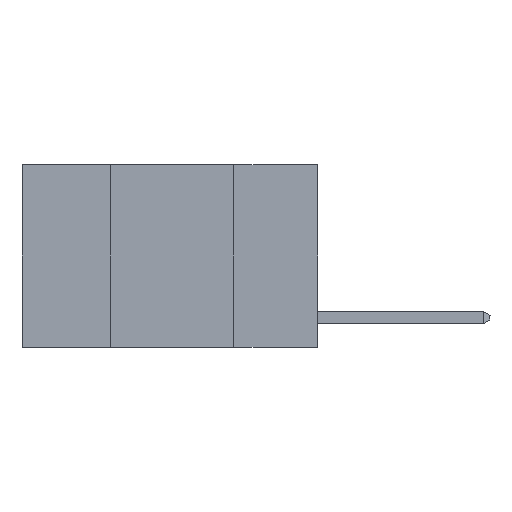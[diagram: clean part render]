
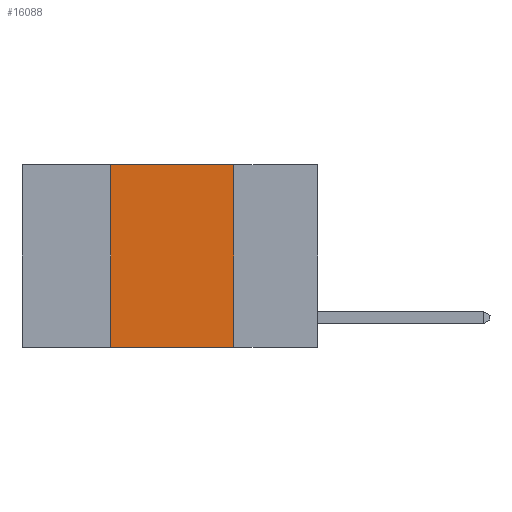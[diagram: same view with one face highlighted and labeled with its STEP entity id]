
A CAD part, left-side view. The second image highlights one B-rep face of the part: STEP entity #16088.
In plain terms, the highlighted planar face has unit normal (-1, 0, 0).
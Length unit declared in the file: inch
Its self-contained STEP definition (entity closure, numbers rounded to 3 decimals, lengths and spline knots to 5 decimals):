
#595 = DIRECTION ( 'NONE',  ( 0., -1., 0. ) ) ;
#1107 = VECTOR ( 'NONE', #4301, 39.37008 ) ;
#1128 = VERTEX_POINT ( 'NONE', #12029 ) ;
#1231 = DIRECTION ( 'NONE',  ( 0., 0., -1. ) ) ;
#1541 = CARTESIAN_POINT ( 'NONE',  ( 0., 0.6, -0.37 ) ) ;
#3491 = AXIS2_PLACEMENT_3D ( 'NONE', #14970, #16253, #1231 ) ;
#4046 = VECTOR ( 'NONE', #595, 39.37008 ) ;
#4301 = DIRECTION ( 'NONE',  ( 0., -1., 0. ) ) ;
#4798 = EDGE_CURVE ( 'NONE', #1128, #5580, #16467, .T. ) ;
#5580 = VERTEX_POINT ( 'NONE', #16965 ) ;
#5707 = EDGE_LOOP ( 'NONE', ( #5910, #8262, #6669, #9400 ) ) ;
#5910 = ORIENTED_EDGE ( 'NONE', *, *, #11385, .F. ) ;
#6521 = DIRECTION ( 'NONE',  ( 0., 0., -1. ) ) ;
#6669 = ORIENTED_EDGE ( 'NONE', *, *, #17532, .F. ) ;
#7467 = LINE ( 'NONE', #8719, #4046 ) ;
#8262 = ORIENTED_EDGE ( 'NONE', *, *, #10761, .F. ) ;
#8719 = CARTESIAN_POINT ( 'NONE',  ( 0., 0.6, 0. ) ) ;
#9289 = CARTESIAN_POINT ( 'NONE',  ( 0., 0.17, 0. ) ) ;
#9400 = ORIENTED_EDGE ( 'NONE', *, *, #4798, .T. ) ;
#10001 = VERTEX_POINT ( 'NONE', #9289 ) ;
#10712 = VERTEX_POINT ( 'NONE', #10860 ) ;
#10761 = EDGE_CURVE ( 'NONE', #10712, #10001, #7467, .T. ) ;
#10860 = CARTESIAN_POINT ( 'NONE',  ( 0., 0.42, 0. ) ) ;
#10956 = FACE_OUTER_BOUND ( 'NONE', #5707, .T. ) ;
#11385 = EDGE_CURVE ( 'NONE', #10001, #5580, #11816, .T. ) ;
#11816 = LINE ( 'NONE', #17541, #15195 ) ;
#12029 = CARTESIAN_POINT ( 'NONE',  ( 0., 0.42, -0.37 ) ) ;
#12073 = CARTESIAN_POINT ( 'NONE',  ( 0., 0.42, 0. ) ) ;
#13455 = PLANE ( 'NONE',  #3491 ) ;
#13484 = DIRECTION ( 'NONE',  ( 0., 0., 1. ) ) ;
#14899 = VECTOR ( 'NONE', #13484, 39.37008 ) ;
#14970 = CARTESIAN_POINT ( 'NONE',  ( 0., 0.6, 0. ) ) ;
#15195 = VECTOR ( 'NONE', #6521, 39.37008 ) ;
#16088 = ADVANCED_FACE ( 'NONE', ( #10956 ), #13455, .F. ) ;
#16253 = DIRECTION ( 'NONE',  ( 1., 0., 0. ) ) ;
#16467 = LINE ( 'NONE', #1541, #1107 ) ;
#16965 = CARTESIAN_POINT ( 'NONE',  ( 0., 0.17, -0.37 ) ) ;
#17307 = LINE ( 'NONE', #12073, #14899 ) ;
#17532 = EDGE_CURVE ( 'NONE', #1128, #10712, #17307, .T. ) ;
#17541 = CARTESIAN_POINT ( 'NONE',  ( 0., 0.17, 0. ) ) ;
